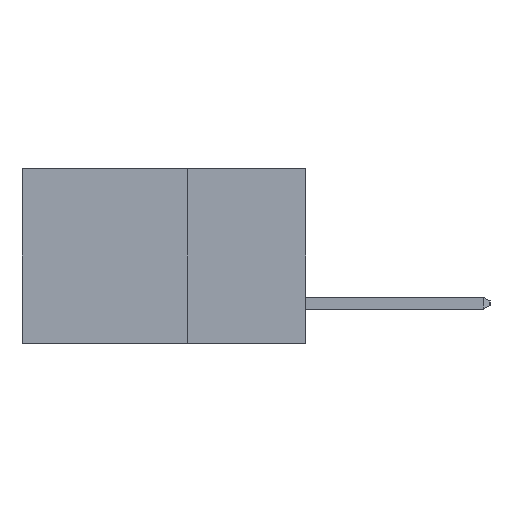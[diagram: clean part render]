
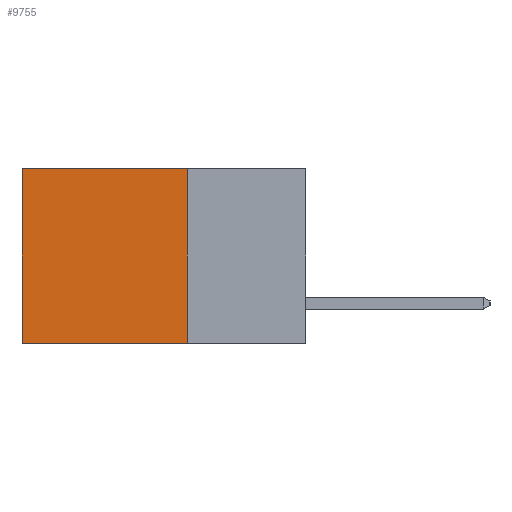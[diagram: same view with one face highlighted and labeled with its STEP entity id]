
A CAD part, left-side view. The second image highlights one B-rep face of the part: STEP entity #9755.
In plain terms, the highlighted planar face has unit normal (-1, 0, 0).
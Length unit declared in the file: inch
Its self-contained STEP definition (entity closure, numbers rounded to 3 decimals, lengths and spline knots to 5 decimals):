
#66 = CARTESIAN_POINT ( 'NONE',  ( 0.298, 0.25, 0. ) ) ;
#1511 = VERTEX_POINT ( 'NONE', #4589 ) ;
#1518 = AXIS2_PLACEMENT_3D ( 'NONE', #4363, #6907, #15360 ) ;
#1863 = CARTESIAN_POINT ( 'NONE',  ( 0.298, 0.25, 0. ) ) ;
#2015 = VECTOR ( 'NONE', #14573, 39.37008 ) ;
#2632 = FACE_OUTER_BOUND ( 'NONE', #15640, .T. ) ;
#3330 = VERTEX_POINT ( 'NONE', #7592 ) ;
#3487 = EDGE_CURVE ( 'NONE', #3330, #1511, #11182, .T. ) ;
#3852 = ORIENTED_EDGE ( 'NONE', *, *, #14416, .F. ) ;
#4127 = LINE ( 'NONE', #13046, #4531 ) ;
#4143 = ORIENTED_EDGE ( 'NONE', *, *, #12718, .F. ) ;
#4363 = CARTESIAN_POINT ( 'NONE',  ( 0.298, 0.25, 0. ) ) ;
#4465 = VERTEX_POINT ( 'NONE', #66 ) ;
#4531 = VECTOR ( 'NONE', #15524, 39.37008 ) ;
#4589 = CARTESIAN_POINT ( 'NONE',  ( 0.298, 0.6, -0.37 ) ) ;
#5708 = EDGE_CURVE ( 'NONE', #4465, #3330, #8311, .T. ) ;
#6539 = ORIENTED_EDGE ( 'NONE', *, *, #5708, .T. ) ;
#6907 = DIRECTION ( 'NONE',  ( 1., 0., 0. ) ) ;
#7219 = CARTESIAN_POINT ( 'NONE',  ( 0.298, 0.25, -0.37 ) ) ;
#7336 = CARTESIAN_POINT ( 'NONE',  ( 0.298, 0.25, 0. ) ) ;
#7592 = CARTESIAN_POINT ( 'NONE',  ( 0.298, 0.6, 0. ) ) ;
#8111 = PLANE ( 'NONE',  #1518 ) ;
#8311 = LINE ( 'NONE', #7336, #2015 ) ;
#8581 = LINE ( 'NONE', #1863, #14620 ) ;
#9750 = ORIENTED_EDGE ( 'NONE', *, *, #3487, .T. ) ;
#9755 = ADVANCED_FACE ( 'NONE', ( #2632 ), #8111, .F. ) ;
#10819 = VECTOR ( 'NONE', #14322, 39.37008 ) ;
#11182 = LINE ( 'NONE', #14378, #10819 ) ;
#11730 = DIRECTION ( 'NONE',  ( 0., 0., -1. ) ) ;
#12091 = VERTEX_POINT ( 'NONE', #7219 ) ;
#12718 = EDGE_CURVE ( 'NONE', #12091, #1511, #4127, .T. ) ;
#13046 = CARTESIAN_POINT ( 'NONE',  ( 0.298, 0.25, -0.37 ) ) ;
#14322 = DIRECTION ( 'NONE',  ( 0., 0., -1. ) ) ;
#14378 = CARTESIAN_POINT ( 'NONE',  ( 0.298, 0.6, 0. ) ) ;
#14416 = EDGE_CURVE ( 'NONE', #4465, #12091, #8581, .T. ) ;
#14573 = DIRECTION ( 'NONE',  ( 0., 1., 0. ) ) ;
#14620 = VECTOR ( 'NONE', #11730, 39.37008 ) ;
#15360 = DIRECTION ( 'NONE',  ( 0., 0., -1. ) ) ;
#15524 = DIRECTION ( 'NONE',  ( 0., 1., 0. ) ) ;
#15640 = EDGE_LOOP ( 'NONE', ( #9750, #4143, #3852, #6539 ) ) ;
